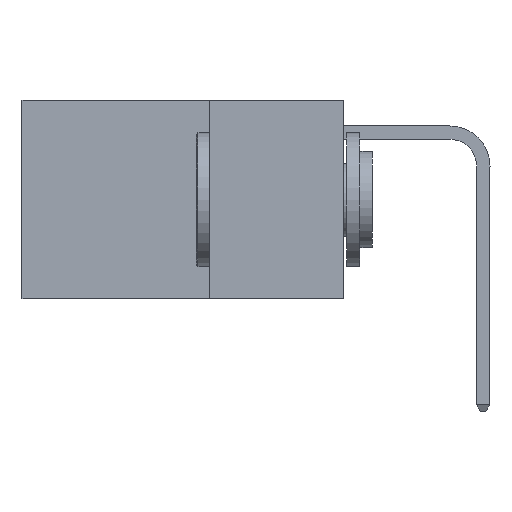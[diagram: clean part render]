
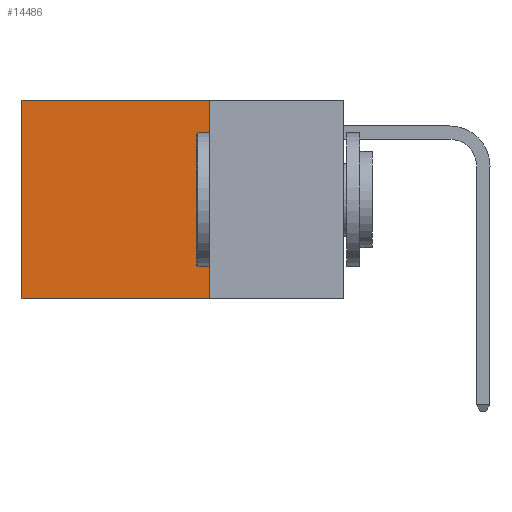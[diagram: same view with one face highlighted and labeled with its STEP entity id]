
A CAD part, left-side view. The second image highlights one B-rep face of the part: STEP entity #14486.
In plain terms, the highlighted planar face has unit normal (-1, 0, 0).
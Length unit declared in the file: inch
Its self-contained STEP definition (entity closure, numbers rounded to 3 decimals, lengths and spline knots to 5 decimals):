
#252 = EDGE_CURVE ( 'NONE', #8922, #11078, #16909, .T. ) ;
#398 = DIRECTION ( 'NONE',  ( 0., 0., -1. ) ) ;
#731 = ORIENTED_EDGE ( 'NONE', *, *, #13483, .T. ) ;
#939 = CARTESIAN_POINT ( 'NONE',  ( 0.2625, 0.25, 0. ) ) ;
#1065 = EDGE_CURVE ( 'NONE', #11531, #11078, #15138, .T. ) ;
#1939 = VECTOR ( 'NONE', #16253, 39.37008 ) ;
#4009 = LINE ( 'NONE', #939, #11989 ) ;
#7114 = ORIENTED_EDGE ( 'NONE', *, *, #252, .T. ) ;
#7292 = ORIENTED_EDGE ( 'NONE', *, *, #14407, .F. ) ;
#7551 = CARTESIAN_POINT ( 'NONE',  ( 0.2625, 0.25, 0. ) ) ;
#8922 = VERTEX_POINT ( 'NONE', #9782 ) ;
#9782 = CARTESIAN_POINT ( 'NONE',  ( 0.2625, 0.6, 0. ) ) ;
#10633 = VERTEX_POINT ( 'NONE', #14747 ) ;
#10749 = DIRECTION ( 'NONE',  ( 0., 0., -1. ) ) ;
#11078 = VERTEX_POINT ( 'NONE', #11219 ) ;
#11210 = ORIENTED_EDGE ( 'NONE', *, *, #1065, .F. ) ;
#11219 = CARTESIAN_POINT ( 'NONE',  ( 0.2625, 0.6, -0.37 ) ) ;
#11531 = VERTEX_POINT ( 'NONE', #20183 ) ;
#11798 = AXIS2_PLACEMENT_3D ( 'NONE', #7551, #20063, #10749 ) ;
#11989 = VECTOR ( 'NONE', #12099, 39.37008 ) ;
#12099 = DIRECTION ( 'NONE',  ( 0., 0., -1. ) ) ;
#12234 = PLANE ( 'NONE',  #11798 ) ;
#13483 = EDGE_CURVE ( 'NONE', #10633, #8922, #18202, .T. ) ;
#14024 = VECTOR ( 'NONE', #17657, 39.37008 ) ;
#14190 = VECTOR ( 'NONE', #398, 39.37008 ) ;
#14407 = EDGE_CURVE ( 'NONE', #10633, #11531, #4009, .T. ) ;
#14486 = ADVANCED_FACE ( 'NONE', ( #18848 ), #12234, .F. ) ;
#14747 = CARTESIAN_POINT ( 'NONE',  ( 0.2625, 0.25, 0. ) ) ;
#15138 = LINE ( 'NONE', #16389, #1939 ) ;
#16078 = CARTESIAN_POINT ( 'NONE',  ( 0.2625, 0.25, 0. ) ) ;
#16253 = DIRECTION ( 'NONE',  ( 0., 1., 0. ) ) ;
#16389 = CARTESIAN_POINT ( 'NONE',  ( 0.2625, 0.25, -0.37 ) ) ;
#16909 = LINE ( 'NONE', #20212, #14190 ) ;
#17657 = DIRECTION ( 'NONE',  ( 0., 1., 0. ) ) ;
#18202 = LINE ( 'NONE', #16078, #14024 ) ;
#18494 = EDGE_LOOP ( 'NONE', ( #7114, #11210, #7292, #731 ) ) ;
#18848 = FACE_OUTER_BOUND ( 'NONE', #18494, .T. ) ;
#20063 = DIRECTION ( 'NONE',  ( 1., 0., 0. ) ) ;
#20183 = CARTESIAN_POINT ( 'NONE',  ( 0.2625, 0.25, -0.37 ) ) ;
#20212 = CARTESIAN_POINT ( 'NONE',  ( 0.2625, 0.6, 0. ) ) ;
